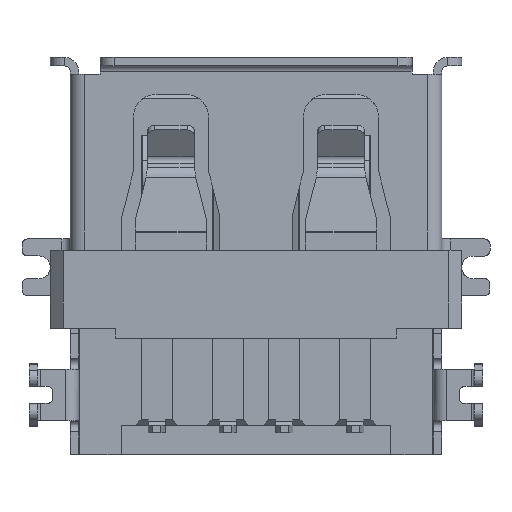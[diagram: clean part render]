
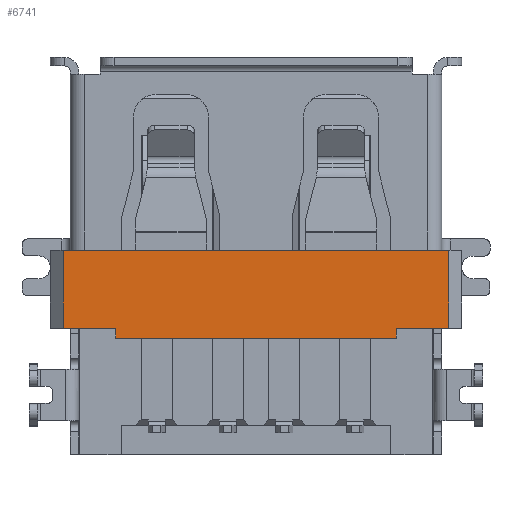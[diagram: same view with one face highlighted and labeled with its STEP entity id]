
A CAD part, front view. The second image highlights one B-rep face of the part: STEP entity #6741.
In plain terms, the highlighted planar face has unit normal (0, -1, 0).
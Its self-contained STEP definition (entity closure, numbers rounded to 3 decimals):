
#528 = EDGE_CURVE ( 'NONE', #22909, #15932, #17676, .T. ) ;
#1059 = VECTOR ( 'NONE', #16892, 1000. ) ;
#1286 = CARTESIAN_POINT ( 'NONE',  ( -0.575, -6.12, 0.83 ) ) ;
#1309 = VERTEX_POINT ( 'NONE', #1979 ) ;
#1979 = CARTESIAN_POINT ( 'NONE',  ( 11.175, -6.12, -0.37 ) ) ;
#2627 = PLANE ( 'NONE',  #26571 ) ;
#2664 = VECTOR ( 'NONE', #19211, 1000. ) ;
#3589 = CARTESIAN_POINT ( 'NONE',  ( 11.175, -6.12, -0.72 ) ) ;
#4036 = CARTESIAN_POINT ( 'NONE',  ( 6.225, -6.12, 2.38 ) ) ;
#4043 = LINE ( 'NONE', #12748, #11496 ) ;
#4061 = ORIENTED_EDGE ( 'NONE', *, *, #23532, .F. ) ;
#5969 = DIRECTION ( 'NONE',  ( 1., 0., 0. ) ) ;
#6009 = EDGE_CURVE ( 'NONE', #22909, #11637, #4043, .T. ) ;
#6487 = CARTESIAN_POINT ( 'NONE',  ( 1.275, -6.12, -0.72 ) ) ;
#6563 = VERTEX_POINT ( 'NONE', #26526 ) ;
#6741 = ADVANCED_FACE ( 'NONE', ( #11327 ), #2627, .F. ) ;
#7037 = DIRECTION ( 'NONE',  ( 0., 0., -1. ) ) ;
#7394 = VERTEX_POINT ( 'NONE', #3589 ) ;
#7882 = CARTESIAN_POINT ( 'NONE',  ( 13.025, -6.12, 2.38 ) ) ;
#8483 = VERTEX_POINT ( 'NONE', #7882 ) ;
#9044 = DIRECTION ( 'NONE',  ( 0., 1., 0. ) ) ;
#9396 = CARTESIAN_POINT ( 'NONE',  ( -0.575, -6.12, 2.38 ) ) ;
#10444 = ORIENTED_EDGE ( 'NONE', *, *, #528, .F. ) ;
#11327 = FACE_OUTER_BOUND ( 'NONE', #12589, .T. ) ;
#11496 = VECTOR ( 'NONE', #28162, 1000. ) ;
#11637 = VERTEX_POINT ( 'NONE', #6487 ) ;
#11852 = DIRECTION ( 'NONE',  ( 0., 0., 1. ) ) ;
#12139 = LINE ( 'NONE', #21153, #12206 ) ;
#12206 = VECTOR ( 'NONE', #7037, 1000. ) ;
#12589 = EDGE_LOOP ( 'NONE', ( #19578, #18937, #10444, #18255, #26570, #27720, #4061, #26731 ) ) ;
#12748 = CARTESIAN_POINT ( 'NONE',  ( 1.275, -6.12, -0.545 ) ) ;
#13270 = EDGE_CURVE ( 'NONE', #15042, #8483, #17446, .T. ) ;
#13647 = VECTOR ( 'NONE', #11852, 1000. ) ;
#14804 = CARTESIAN_POINT ( 'NONE',  ( 6.225, -6.12, -0.72 ) ) ;
#14934 = LINE ( 'NONE', #14804, #2664 ) ;
#15025 = DIRECTION ( 'NONE',  ( 0., 0., -1. ) ) ;
#15042 = VERTEX_POINT ( 'NONE', #9396 ) ;
#15393 = DIRECTION ( 'NONE',  ( -1., 0., 0. ) ) ;
#15911 = VECTOR ( 'NONE', #15025, 1000. ) ;
#15932 = VERTEX_POINT ( 'NONE', #18041 ) ;
#16230 = LINE ( 'NONE', #27069, #17931 ) ;
#16892 = DIRECTION ( 'NONE',  ( 1., 0., 0. ) ) ;
#17446 = LINE ( 'NONE', #4036, #1059 ) ;
#17676 = LINE ( 'NONE', #17956, #21441 ) ;
#17750 = EDGE_CURVE ( 'NONE', #7394, #11637, #14934, .T. ) ;
#17931 = VECTOR ( 'NONE', #26644, 1000. ) ;
#17956 = CARTESIAN_POINT ( 'NONE',  ( 6.225, -6.12, -0.37 ) ) ;
#18041 = CARTESIAN_POINT ( 'NONE',  ( -0.575, -6.12, -0.37 ) ) ;
#18140 = EDGE_CURVE ( 'NONE', #1309, #7394, #19585, .T. ) ;
#18255 = ORIENTED_EDGE ( 'NONE', *, *, #6009, .T. ) ;
#18455 = EDGE_CURVE ( 'NONE', #15932, #15042, #18717, .T. ) ;
#18717 = LINE ( 'NONE', #1286, #13647 ) ;
#18937 = ORIENTED_EDGE ( 'NONE', *, *, #18455, .F. ) ;
#19211 = DIRECTION ( 'NONE',  ( -1., 0., 0. ) ) ;
#19317 = CARTESIAN_POINT ( 'NONE',  ( 11.175, -6.12, -0.545 ) ) ;
#19441 = CARTESIAN_POINT ( 'NONE',  ( 1.275, -6.12, -0.37 ) ) ;
#19578 = ORIENTED_EDGE ( 'NONE', *, *, #13270, .F. ) ;
#19585 = LINE ( 'NONE', #19317, #15911 ) ;
#19962 = EDGE_CURVE ( 'NONE', #8483, #6563, #12139, .T. ) ;
#21153 = CARTESIAN_POINT ( 'NONE',  ( 13.025, -6.12, 0.83 ) ) ;
#21441 = VECTOR ( 'NONE', #15393, 1000. ) ;
#22909 = VERTEX_POINT ( 'NONE', #19441 ) ;
#23532 = EDGE_CURVE ( 'NONE', #6563, #1309, #16230, .T. ) ;
#24316 = CARTESIAN_POINT ( 'NONE',  ( 6.225, -6.12, 0.83 ) ) ;
#26526 = CARTESIAN_POINT ( 'NONE',  ( 13.025, -6.12, -0.37 ) ) ;
#26570 = ORIENTED_EDGE ( 'NONE', *, *, #17750, .F. ) ;
#26571 = AXIS2_PLACEMENT_3D ( 'NONE', #24316, #9044, #5969 ) ;
#26644 = DIRECTION ( 'NONE',  ( -1., 0., 0. ) ) ;
#26731 = ORIENTED_EDGE ( 'NONE', *, *, #19962, .F. ) ;
#27069 = CARTESIAN_POINT ( 'NONE',  ( 6.225, -6.12, -0.37 ) ) ;
#27720 = ORIENTED_EDGE ( 'NONE', *, *, #18140, .F. ) ;
#28162 = DIRECTION ( 'NONE',  ( 0., 0., -1. ) ) ;
